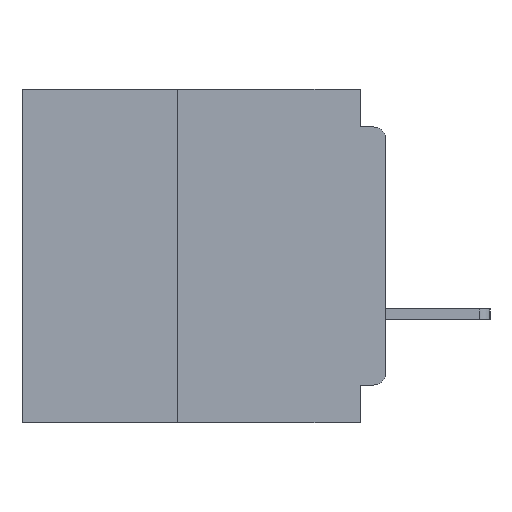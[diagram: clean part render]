
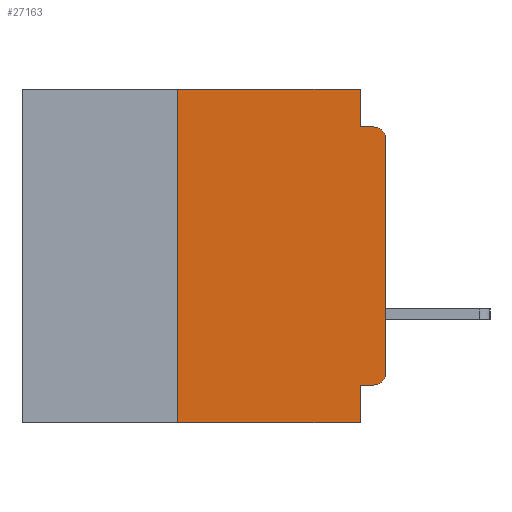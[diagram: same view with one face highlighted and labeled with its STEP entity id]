
A CAD part, left-side view. The second image highlights one B-rep face of the part: STEP entity #27163.
In plain terms, the highlighted planar face has unit normal (-1, 0, 0).
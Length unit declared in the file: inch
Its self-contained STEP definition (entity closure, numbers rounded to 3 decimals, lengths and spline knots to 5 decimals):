
#241 = LINE ( 'NONE', #27756, #6850 ) ;
#664 = EDGE_CURVE ( 'NONE', #21323, #4394, #7295, .T. ) ;
#1034 = VECTOR ( 'NONE', #26866, 39.37008 ) ;
#1080 = EDGE_CURVE ( 'NONE', #21659, #23533, #7254, .T. ) ;
#1233 = EDGE_CURVE ( 'NONE', #1381, #34041, #8534, .T. ) ;
#1381 = VERTEX_POINT ( 'NONE', #28858 ) ;
#1395 = ORIENTED_EDGE ( 'NONE', *, *, #1080, .F. ) ;
#1560 = DIRECTION ( 'NONE',  ( 0., 0., 1. ) ) ;
#1568 = VECTOR ( 'NONE', #9723, 39.37008 ) ;
#1697 = DIRECTION ( 'NONE',  ( 0., 0., -1. ) ) ;
#2868 = AXIS2_PLACEMENT_3D ( 'NONE', #19318, #11619, #11583 ) ;
#3201 = ORIENTED_EDGE ( 'NONE', *, *, #16128, .F. ) ;
#3458 = DIRECTION ( 'NONE',  ( 0., 0., -1. ) ) ;
#4394 = VERTEX_POINT ( 'NONE', #30669 ) ;
#4880 = CARTESIAN_POINT ( 'NONE',  ( 0., 0.015, -0.045 ) ) ;
#6746 = EDGE_CURVE ( 'NONE', #21323, #1381, #241, .T. ) ;
#6850 = VECTOR ( 'NONE', #24996, 39.37008 ) ;
#7254 = LINE ( 'NONE', #15030, #21109 ) ;
#7295 = CIRCLE ( 'NONE', #2868, 0.015 ) ;
#7589 = CARTESIAN_POINT ( 'NONE',  ( 0., 0.031, -0.4 ) ) ;
#8350 = CARTESIAN_POINT ( 'NONE',  ( 0., 0.031, 0. ) ) ;
#8521 = EDGE_CURVE ( 'NONE', #31724, #13408, #31767, .T. ) ;
#8534 = LINE ( 'NONE', #7589, #1034 ) ;
#9246 = VERTEX_POINT ( 'NONE', #27064 ) ;
#9723 = DIRECTION ( 'NONE',  ( 0., 0., 1. ) ) ;
#10503 = EDGE_CURVE ( 'NONE', #9246, #16241, #16415, .T. ) ;
#11583 = DIRECTION ( 'NONE',  ( 0., 0., -1. ) ) ;
#11619 = DIRECTION ( 'NONE',  ( -1., 0., 0. ) ) ;
#13130 = DIRECTION ( 'NONE',  ( 1., 0., 0. ) ) ;
#13191 = ORIENTED_EDGE ( 'NONE', *, *, #1233, .F. ) ;
#13408 = VERTEX_POINT ( 'NONE', #4880 ) ;
#13623 = ORIENTED_EDGE ( 'NONE', *, *, #8521, .T. ) ;
#14971 = ORIENTED_EDGE ( 'NONE', *, *, #6746, .F. ) ;
#15030 = CARTESIAN_POINT ( 'NONE',  ( 0., 0.031, 0. ) ) ;
#15376 = ORIENTED_EDGE ( 'NONE', *, *, #35597, .F. ) ;
#16120 = VECTOR ( 'NONE', #16625, 39.37008 ) ;
#16128 = EDGE_CURVE ( 'NONE', #16241, #21659, #25983, .T. ) ;
#16241 = VERTEX_POINT ( 'NONE', #26074 ) ;
#16415 = LINE ( 'NONE', #29104, #1568 ) ;
#16625 = DIRECTION ( 'NONE',  ( 0., -1., 0. ) ) ;
#16736 = FACE_OUTER_BOUND ( 'NONE', #27531, .T. ) ;
#16918 = VECTOR ( 'NONE', #1560, 39.37008 ) ;
#17028 = LINE ( 'NONE', #19408, #16120 ) ;
#17126 = CARTESIAN_POINT ( 'NONE',  ( 0., 0.437, 0. ) ) ;
#17407 = DIRECTION ( 'NONE',  ( 0., -1., 0. ) ) ;
#18255 = LINE ( 'NONE', #25765, #23521 ) ;
#18396 = DIRECTION ( 'NONE',  ( -1., 0., 0. ) ) ;
#18601 = VECTOR ( 'NONE', #25598, 39.37008 ) ;
#19318 = CARTESIAN_POINT ( 'NONE',  ( 0., 0.015, -0.34 ) ) ;
#19408 = CARTESIAN_POINT ( 'NONE',  ( 0., 0.437, -0.4 ) ) ;
#19867 = EDGE_CURVE ( 'NONE', #9246, #34041, #17028, .T. ) ;
#20133 = ORIENTED_EDGE ( 'NONE', *, *, #24919, .T. ) ;
#21109 = VECTOR ( 'NONE', #3458, 39.37008 ) ;
#21323 = VERTEX_POINT ( 'NONE', #26298 ) ;
#21659 = VERTEX_POINT ( 'NONE', #8350 ) ;
#22045 = AXIS2_PLACEMENT_3D ( 'NONE', #29735, #13130, #32432 ) ;
#22643 = AXIS2_PLACEMENT_3D ( 'NONE', #34862, #18396, #1697 ) ;
#23521 = VECTOR ( 'NONE', #17407, 39.37008 ) ;
#23533 = VERTEX_POINT ( 'NONE', #28090 ) ;
#24276 = LINE ( 'NONE', #31993, #16918 ) ;
#24919 = EDGE_CURVE ( 'NONE', #4394, #31724, #24276, .T. ) ;
#24996 = DIRECTION ( 'NONE',  ( 0., 1., 0. ) ) ;
#25128 = CARTESIAN_POINT ( 'NONE',  ( 0., 0.031, -0.4 ) ) ;
#25384 = ORIENTED_EDGE ( 'NONE', *, *, #10503, .F. ) ;
#25598 = DIRECTION ( 'NONE',  ( 0., -1., 0. ) ) ;
#25765 = CARTESIAN_POINT ( 'NONE',  ( 0., 0., -0.045 ) ) ;
#25983 = LINE ( 'NONE', #17126, #18601 ) ;
#26074 = CARTESIAN_POINT ( 'NONE',  ( 0., 0.25, 0. ) ) ;
#26298 = CARTESIAN_POINT ( 'NONE',  ( 0., 0.015, -0.355 ) ) ;
#26866 = DIRECTION ( 'NONE',  ( 0., 0., -1. ) ) ;
#27064 = CARTESIAN_POINT ( 'NONE',  ( 0., 0.25, -0.4 ) ) ;
#27163 = ADVANCED_FACE ( 'NONE', ( #16736 ), #32214, .F. ) ;
#27531 = EDGE_LOOP ( 'NONE', ( #20133, #13623, #15376, #1395, #3201, #25384, #34337, #13191, #14971, #29682 ) ) ;
#27756 = CARTESIAN_POINT ( 'NONE',  ( 0., 0., -0.355 ) ) ;
#28090 = CARTESIAN_POINT ( 'NONE',  ( 0., 0.031, -0.045 ) ) ;
#28858 = CARTESIAN_POINT ( 'NONE',  ( 0., 0.031, -0.355 ) ) ;
#29104 = CARTESIAN_POINT ( 'NONE',  ( 0., 0.25, -0.4 ) ) ;
#29682 = ORIENTED_EDGE ( 'NONE', *, *, #664, .T. ) ;
#29735 = CARTESIAN_POINT ( 'NONE',  ( 0., 0.437, 0. ) ) ;
#30669 = CARTESIAN_POINT ( 'NONE',  ( 0., 0., -0.34 ) ) ;
#31724 = VERTEX_POINT ( 'NONE', #34347 ) ;
#31767 = CIRCLE ( 'NONE', #22643, 0.015 ) ;
#31993 = CARTESIAN_POINT ( 'NONE',  ( 0., 0., 0. ) ) ;
#32214 = PLANE ( 'NONE',  #22045 ) ;
#32432 = DIRECTION ( 'NONE',  ( 0., 0., -1. ) ) ;
#34041 = VERTEX_POINT ( 'NONE', #25128 ) ;
#34337 = ORIENTED_EDGE ( 'NONE', *, *, #19867, .T. ) ;
#34347 = CARTESIAN_POINT ( 'NONE',  ( 0., 0., -0.06 ) ) ;
#34862 = CARTESIAN_POINT ( 'NONE',  ( 0., 0.015, -0.06 ) ) ;
#35597 = EDGE_CURVE ( 'NONE', #23533, #13408, #18255, .T. ) ;
